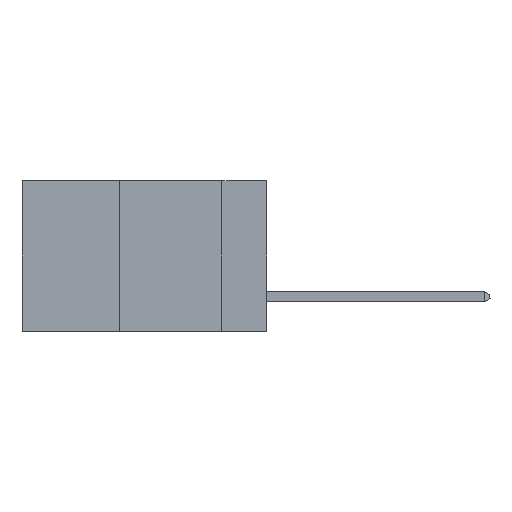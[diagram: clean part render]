
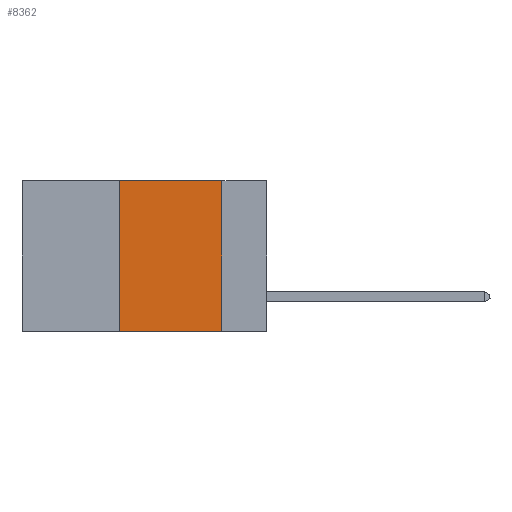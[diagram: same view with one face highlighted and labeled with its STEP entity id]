
A CAD part, left-side view. The second image highlights one B-rep face of the part: STEP entity #8362.
In plain terms, the highlighted planar face has unit normal (-1, 0, 0).
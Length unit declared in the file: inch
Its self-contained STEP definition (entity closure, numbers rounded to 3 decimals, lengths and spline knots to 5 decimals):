
#149 = CARTESIAN_POINT ( 'NONE',  ( 0., 0.6, 0. ) ) ;
#354 = LINE ( 'NONE', #12632, #9932 ) ;
#1284 = DIRECTION ( 'NONE',  ( 0., 0., 1. ) ) ;
#1313 = DIRECTION ( 'NONE',  ( 1., 0., 0. ) ) ;
#1362 = VERTEX_POINT ( 'NONE', #6727 ) ;
#1503 = DIRECTION ( 'NONE',  ( 0., 0., -1. ) ) ;
#2300 = DIRECTION ( 'NONE',  ( 0., -1., 0. ) ) ;
#2360 = VECTOR ( 'NONE', #1284, 39.37008 ) ;
#2787 = VERTEX_POINT ( 'NONE', #13105 ) ;
#2819 = FACE_OUTER_BOUND ( 'NONE', #11277, .T. ) ;
#2954 = CARTESIAN_POINT ( 'NONE',  ( 0., 0.6, 0. ) ) ;
#4452 = VERTEX_POINT ( 'NONE', #9587 ) ;
#4489 = EDGE_CURVE ( 'NONE', #2787, #7134, #354, .T. ) ;
#4490 = PLANE ( 'NONE',  #10673 ) ;
#4913 = CARTESIAN_POINT ( 'NONE',  ( 0., 0.36, 0. ) ) ;
#4972 = CARTESIAN_POINT ( 'NONE',  ( 0., 0.11, -0.37 ) ) ;
#6261 = DIRECTION ( 'NONE',  ( 0., -1., 0. ) ) ;
#6727 = CARTESIAN_POINT ( 'NONE',  ( 0., 0.36, -0.37 ) ) ;
#7067 = EDGE_CURVE ( 'NONE', #1362, #7134, #7720, .T. ) ;
#7134 = VERTEX_POINT ( 'NONE', #4972 ) ;
#7472 = ORIENTED_EDGE ( 'NONE', *, *, #12044, .F. ) ;
#7570 = VECTOR ( 'NONE', #6261, 39.37008 ) ;
#7720 = LINE ( 'NONE', #8904, #14024 ) ;
#8224 = LINE ( 'NONE', #4913, #2360 ) ;
#8362 = ADVANCED_FACE ( 'NONE', ( #2819 ), #4490, .F. ) ;
#8904 = CARTESIAN_POINT ( 'NONE',  ( 0., 0.6, -0.37 ) ) ;
#9587 = CARTESIAN_POINT ( 'NONE',  ( 0., 0.36, 0. ) ) ;
#9818 = ORIENTED_EDGE ( 'NONE', *, *, #10134, .F. ) ;
#9932 = VECTOR ( 'NONE', #1503, 39.37008 ) ;
#10134 = EDGE_CURVE ( 'NONE', #4452, #2787, #13498, .T. ) ;
#10673 = AXIS2_PLACEMENT_3D ( 'NONE', #149, #1313, #12352 ) ;
#11277 = EDGE_LOOP ( 'NONE', ( #14063, #9818, #7472, #12898 ) ) ;
#12044 = EDGE_CURVE ( 'NONE', #1362, #4452, #8224, .T. ) ;
#12352 = DIRECTION ( 'NONE',  ( 0., 0., -1. ) ) ;
#12632 = CARTESIAN_POINT ( 'NONE',  ( 0., 0.11, 0. ) ) ;
#12898 = ORIENTED_EDGE ( 'NONE', *, *, #7067, .T. ) ;
#13105 = CARTESIAN_POINT ( 'NONE',  ( 0., 0.11, 0. ) ) ;
#13498 = LINE ( 'NONE', #2954, #7570 ) ;
#14024 = VECTOR ( 'NONE', #2300, 39.37008 ) ;
#14063 = ORIENTED_EDGE ( 'NONE', *, *, #4489, .F. ) ;
